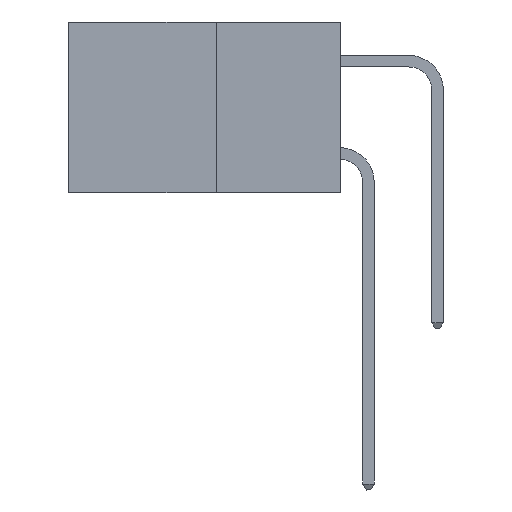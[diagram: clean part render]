
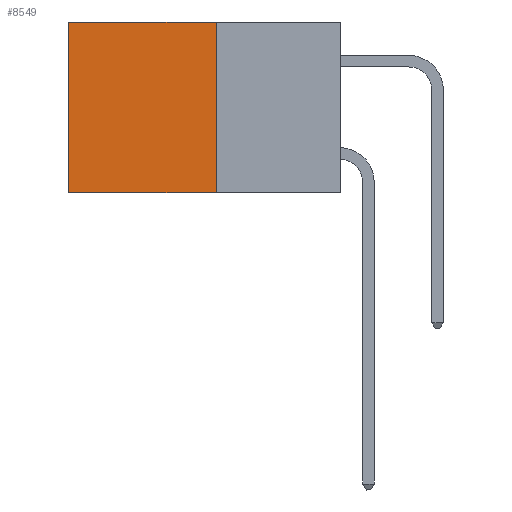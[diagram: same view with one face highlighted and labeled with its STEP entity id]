
A CAD part, left-side view. The second image highlights one B-rep face of the part: STEP entity #8549.
In plain terms, the highlighted planar face has unit normal (-1, 0, 0).
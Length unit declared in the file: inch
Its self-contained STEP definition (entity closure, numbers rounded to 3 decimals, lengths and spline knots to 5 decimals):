
#394 = DIRECTION ( 'NONE',  ( 0., 0., -1. ) ) ;
#1356 = VERTEX_POINT ( 'NONE', #6200 ) ;
#2514 = EDGE_CURVE ( 'NONE', #13519, #6193, #28243, .T. ) ;
#3278 = CARTESIAN_POINT ( 'NONE',  ( 0.277, 0.27, -0.37 ) ) ;
#3474 = DIRECTION ( 'NONE',  ( 0., 0., -1. ) ) ;
#4376 = CARTESIAN_POINT ( 'NONE',  ( 0.277, 0.27, -0.37 ) ) ;
#5688 = VECTOR ( 'NONE', #19805, 39.37008 ) ;
#6193 = VERTEX_POINT ( 'NONE', #18149 ) ;
#6200 = CARTESIAN_POINT ( 'NONE',  ( 0.277, 0.27, 0. ) ) ;
#8549 = ADVANCED_FACE ( 'NONE', ( #9968 ), #9655, .F. ) ;
#8590 = LINE ( 'NONE', #11226, #19892 ) ;
#8739 = ORIENTED_EDGE ( 'NONE', *, *, #17399, .F. ) ;
#9655 = PLANE ( 'NONE',  #25146 ) ;
#9968 = FACE_OUTER_BOUND ( 'NONE', #29012, .T. ) ;
#11226 = CARTESIAN_POINT ( 'NONE',  ( 0.277, 0.27, -0.37 ) ) ;
#11903 = ORIENTED_EDGE ( 'NONE', *, *, #2514, .F. ) ;
#12361 = CARTESIAN_POINT ( 'NONE',  ( 0.277, 0.59, 0. ) ) ;
#13299 = EDGE_CURVE ( 'NONE', #15857, #6193, #16925, .T. ) ;
#13445 = DIRECTION ( 'NONE',  ( 0., 0., -1. ) ) ;
#13519 = VERTEX_POINT ( 'NONE', #4376 ) ;
#14140 = DIRECTION ( 'NONE',  ( 1., 0., 0. ) ) ;
#14845 = CARTESIAN_POINT ( 'NONE',  ( 0.277, 0.59, -0.37 ) ) ;
#15857 = VERTEX_POINT ( 'NONE', #12361 ) ;
#16925 = LINE ( 'NONE', #14845, #22213 ) ;
#17399 = EDGE_CURVE ( 'NONE', #1356, #13519, #8590, .T. ) ;
#17531 = CARTESIAN_POINT ( 'NONE',  ( 0.277, 0.27, 0. ) ) ;
#17761 = LINE ( 'NONE', #17531, #5688 ) ;
#18149 = CARTESIAN_POINT ( 'NONE',  ( 0.277, 0.59, -0.37 ) ) ;
#19805 = DIRECTION ( 'NONE',  ( 0., 1., 0. ) ) ;
#19892 = VECTOR ( 'NONE', #13445, 39.37008 ) ;
#22213 = VECTOR ( 'NONE', #3474, 39.37008 ) ;
#23431 = ORIENTED_EDGE ( 'NONE', *, *, #13299, .T. ) ;
#23432 = DIRECTION ( 'NONE',  ( 0., 1., 0. ) ) ;
#23491 = ORIENTED_EDGE ( 'NONE', *, *, #24294, .T. ) ;
#24294 = EDGE_CURVE ( 'NONE', #1356, #15857, #17761, .T. ) ;
#25146 = AXIS2_PLACEMENT_3D ( 'NONE', #27647, #14140, #394 ) ;
#27548 = VECTOR ( 'NONE', #23432, 39.37008 ) ;
#27647 = CARTESIAN_POINT ( 'NONE',  ( 0.277, 0.27, -0.37 ) ) ;
#28243 = LINE ( 'NONE', #3278, #27548 ) ;
#29012 = EDGE_LOOP ( 'NONE', ( #23431, #11903, #8739, #23491 ) ) ;
